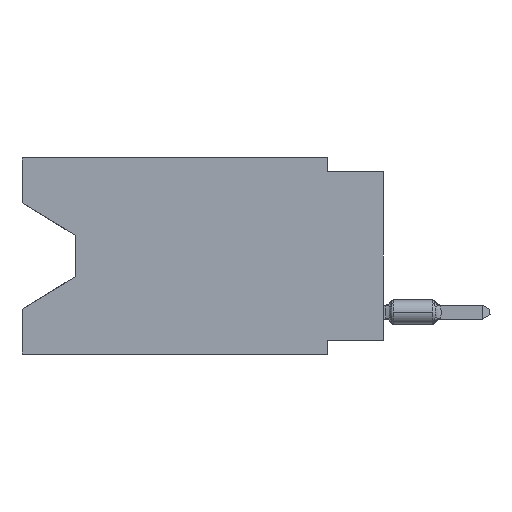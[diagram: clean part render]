
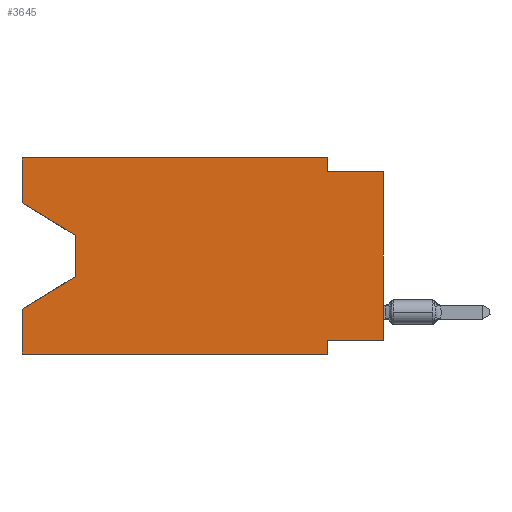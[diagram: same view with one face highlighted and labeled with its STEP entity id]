
A CAD part, left-side view. The second image highlights one B-rep face of the part: STEP entity #3645.
In plain terms, the highlighted planar face has unit normal (-1, 0, 0).
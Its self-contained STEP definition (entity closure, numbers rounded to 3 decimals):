
#1639 = CARTESIAN_POINT ( 'NONE',  ( 0., 2.54, -8.89 ) ) ;
#1700 = VECTOR ( 'NONE', #26946, 1000. ) ;
#2845 = DIRECTION ( 'NONE',  ( 0., -1., 0. ) ) ;
#3621 = VERTEX_POINT ( 'NONE', #17680 ) ;
#3645 = ADVANCED_FACE ( 'NONE', ( #4158 ), #15304, .F. ) ;
#4158 = FACE_OUTER_BOUND ( 'NONE', #5215, .T. ) ;
#4336 = EDGE_CURVE ( 'NONE', #28523, #22751, #7381, .T. ) ;
#4534 = ORIENTED_EDGE ( 'NONE', *, *, #33775, .F. ) ;
#4537 = ORIENTED_EDGE ( 'NONE', *, *, #5888, .T. ) ;
#5045 = VECTOR ( 'NONE', #6150, 1000. ) ;
#5106 = VERTEX_POINT ( 'NONE', #7008 ) ;
#5215 = EDGE_LOOP ( 'NONE', ( #13162, #4537, #13864, #19976, #17152, #18586, #8410, #19072, #33840, #4534, #23698, #18810 ) ) ;
#5888 = EDGE_CURVE ( 'NONE', #17460, #21572, #31137, .T. ) ;
#6150 = DIRECTION ( 'NONE',  ( 0., 0., -1. ) ) ;
#6761 = EDGE_CURVE ( 'NONE', #3621, #24419, #29006, .T. ) ;
#6914 = CARTESIAN_POINT ( 'NONE',  ( 0., 16.383, 0. ) ) ;
#7008 = CARTESIAN_POINT ( 'NONE',  ( 0., 16.383, 0. ) ) ;
#7198 = CARTESIAN_POINT ( 'NONE',  ( 0., 16.383, 0. ) ) ;
#7381 = LINE ( 'NONE', #7198, #35308 ) ;
#7496 = DIRECTION ( 'NONE',  ( 0., 0., 1. ) ) ;
#7531 = CARTESIAN_POINT ( 'NONE',  ( 0., 0., -0.635 ) ) ;
#8111 = LINE ( 'NONE', #22346, #24771 ) ;
#8410 = ORIENTED_EDGE ( 'NONE', *, *, #30908, .F. ) ;
#9401 = CARTESIAN_POINT ( 'NONE',  ( 0., 16.383, -8.89 ) ) ;
#9552 = CARTESIAN_POINT ( 'NONE',  ( 0., 13.97, -5.385 ) ) ;
#10625 = VECTOR ( 'NONE', #17638, 1000. ) ;
#11328 = LINE ( 'NONE', #33404, #27307 ) ;
#11608 = LINE ( 'NONE', #9401, #10625 ) ;
#12171 = EDGE_CURVE ( 'NONE', #33611, #17460, #8111, .T. ) ;
#12563 = LINE ( 'NONE', #15833, #1700 ) ;
#12637 = CARTESIAN_POINT ( 'NONE',  ( 0., 0., -8.255 ) ) ;
#13162 = ORIENTED_EDGE ( 'NONE', *, *, #12171, .T. ) ;
#13864 = ORIENTED_EDGE ( 'NONE', *, *, #20635, .T. ) ;
#15292 = VERTEX_POINT ( 'NONE', #21328 ) ;
#15304 = PLANE ( 'NONE',  #28364 ) ;
#15833 = CARTESIAN_POINT ( 'NONE',  ( 0., 2.54, 0. ) ) ;
#16023 = EDGE_CURVE ( 'NONE', #15292, #29267, #16725, .T. ) ;
#16144 = EDGE_CURVE ( 'NONE', #28523, #24419, #11608, .T. ) ;
#16725 = LINE ( 'NONE', #27844, #26252 ) ;
#17152 = ORIENTED_EDGE ( 'NONE', *, *, #16144, .T. ) ;
#17306 = CARTESIAN_POINT ( 'NONE',  ( 0., 13.97, -3.505 ) ) ;
#17460 = VERTEX_POINT ( 'NONE', #24348 ) ;
#17612 = VERTEX_POINT ( 'NONE', #28154 ) ;
#17638 = DIRECTION ( 'NONE',  ( 0., -1., 0. ) ) ;
#17680 = CARTESIAN_POINT ( 'NONE',  ( 0., 2.54, -8.255 ) ) ;
#17883 = VECTOR ( 'NONE', #7496, 1000. ) ;
#18397 = VECTOR ( 'NONE', #20160, 1000. ) ;
#18411 = LINE ( 'NONE', #6914, #34397 ) ;
#18586 = ORIENTED_EDGE ( 'NONE', *, *, #6761, .F. ) ;
#18810 = ORIENTED_EDGE ( 'NONE', *, *, #23247, .F. ) ;
#19072 = ORIENTED_EDGE ( 'NONE', *, *, #33199, .T. ) ;
#19572 = CARTESIAN_POINT ( 'NONE',  ( 0., 13.97, -5.385 ) ) ;
#19976 = ORIENTED_EDGE ( 'NONE', *, *, #4336, .F. ) ;
#20043 = CARTESIAN_POINT ( 'NONE',  ( 0., 16.383, -2.038 ) ) ;
#20160 = DIRECTION ( 'NONE',  ( 0., 0.855, -0.519 ) ) ;
#20471 = CARTESIAN_POINT ( 'NONE',  ( 0., 16.383, -8.89 ) ) ;
#20590 = DIRECTION ( 'NONE',  ( 1., 0., 0. ) ) ;
#20635 = EDGE_CURVE ( 'NONE', #21572, #22751, #28722, .T. ) ;
#21328 = CARTESIAN_POINT ( 'NONE',  ( 0., 2.54, -0.635 ) ) ;
#21383 = LINE ( 'NONE', #32502, #17883 ) ;
#21572 = VERTEX_POINT ( 'NONE', #19572 ) ;
#22346 = CARTESIAN_POINT ( 'NONE',  ( 0., 16.383, -2.038 ) ) ;
#22751 = VERTEX_POINT ( 'NONE', #29793 ) ;
#22809 = CARTESIAN_POINT ( 'NONE',  ( 0., 2.54, -8.89 ) ) ;
#23247 = EDGE_CURVE ( 'NONE', #33611, #5106, #21383, .T. ) ;
#23530 = DIRECTION ( 'NONE',  ( 0., 0., -1. ) ) ;
#23698 = ORIENTED_EDGE ( 'NONE', *, *, #34842, .F. ) ;
#23734 = DIRECTION ( 'NONE',  ( 0., 1., 0. ) ) ;
#24342 = DIRECTION ( 'NONE',  ( 0., 0., 1. ) ) ;
#24348 = CARTESIAN_POINT ( 'NONE',  ( 0., 13.97, -3.505 ) ) ;
#24419 = VERTEX_POINT ( 'NONE', #22809 ) ;
#24771 = VECTOR ( 'NONE', #33474, 1000. ) ;
#26252 = VECTOR ( 'NONE', #2845, 1000. ) ;
#26406 = DIRECTION ( 'NONE',  ( 0., 0., -1. ) ) ;
#26946 = DIRECTION ( 'NONE',  ( 0., 0., -1. ) ) ;
#27254 = VECTOR ( 'NONE', #23530, 1000. ) ;
#27307 = VECTOR ( 'NONE', #29621, 1000. ) ;
#27844 = CARTESIAN_POINT ( 'NONE',  ( 0., 0., -0.635 ) ) ;
#28154 = CARTESIAN_POINT ( 'NONE',  ( 0., 0., -8.255 ) ) ;
#28364 = AXIS2_PLACEMENT_3D ( 'NONE', #31705, #20590, #26406 ) ;
#28523 = VERTEX_POINT ( 'NONE', #20471 ) ;
#28722 = LINE ( 'NONE', #9552, #18397 ) ;
#29006 = LINE ( 'NONE', #1639, #27254 ) ;
#29267 = VERTEX_POINT ( 'NONE', #7531 ) ;
#29621 = DIRECTION ( 'NONE',  ( 0., 0., 1. ) ) ;
#29793 = CARTESIAN_POINT ( 'NONE',  ( 0., 16.383, -6.852 ) ) ;
#29931 = VERTEX_POINT ( 'NONE', #33744 ) ;
#30289 = VECTOR ( 'NONE', #23734, 1000. ) ;
#30908 = EDGE_CURVE ( 'NONE', #17612, #3621, #31768, .T. ) ;
#31137 = LINE ( 'NONE', #17306, #5045 ) ;
#31705 = CARTESIAN_POINT ( 'NONE',  ( 0., 16.383, 0. ) ) ;
#31768 = LINE ( 'NONE', #12637, #30289 ) ;
#32502 = CARTESIAN_POINT ( 'NONE',  ( 0., 16.383, 0. ) ) ;
#33199 = EDGE_CURVE ( 'NONE', #17612, #29267, #11328, .T. ) ;
#33404 = CARTESIAN_POINT ( 'NONE',  ( 0., 0., 0. ) ) ;
#33474 = DIRECTION ( 'NONE',  ( 0., -0.855, -0.519 ) ) ;
#33611 = VERTEX_POINT ( 'NONE', #20043 ) ;
#33744 = CARTESIAN_POINT ( 'NONE',  ( 0., 2.54, 0. ) ) ;
#33775 = EDGE_CURVE ( 'NONE', #29931, #15292, #12563, .T. ) ;
#33840 = ORIENTED_EDGE ( 'NONE', *, *, #16023, .F. ) ;
#34397 = VECTOR ( 'NONE', #34827, 1000. ) ;
#34827 = DIRECTION ( 'NONE',  ( 0., -1., 0. ) ) ;
#34842 = EDGE_CURVE ( 'NONE', #5106, #29931, #18411, .T. ) ;
#35308 = VECTOR ( 'NONE', #24342, 1000. ) ;
